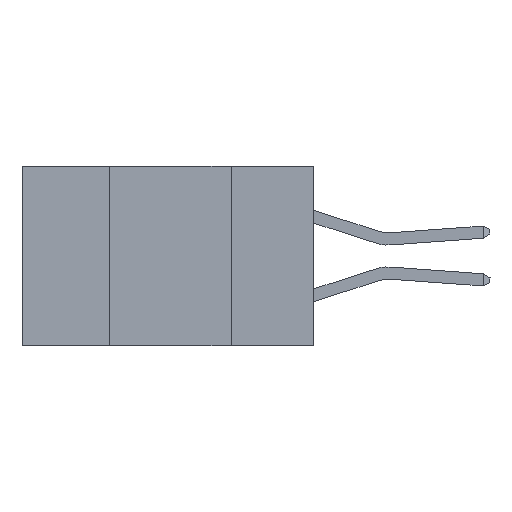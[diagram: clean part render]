
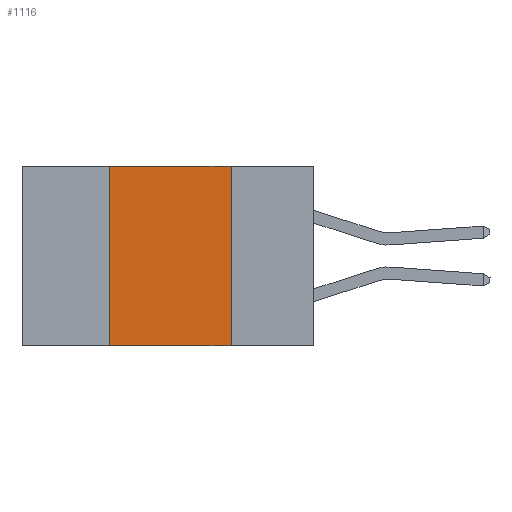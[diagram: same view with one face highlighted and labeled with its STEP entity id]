
A CAD part, left-side view. The second image highlights one B-rep face of the part: STEP entity #1116.
In plain terms, the highlighted planar face has unit normal (-1, 0, 0).
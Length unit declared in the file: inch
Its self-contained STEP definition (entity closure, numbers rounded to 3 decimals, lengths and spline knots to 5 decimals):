
#257 = VERTEX_POINT ( 'NONE', #1028 ) ;
#342 = DIRECTION ( 'NONE',  ( 0., 0., -1. ) ) ;
#811 = FACE_OUTER_BOUND ( 'NONE', #4096, .T. ) ;
#956 = CARTESIAN_POINT ( 'NONE',  ( 0., 0.17, 0. ) ) ;
#1028 = CARTESIAN_POINT ( 'NONE',  ( 0., 0.42, -0.37 ) ) ;
#1116 = ADVANCED_FACE ( 'NONE', ( #811 ), #3273, .F. ) ;
#1811 = VECTOR ( 'NONE', #8453, 39.37008 ) ;
#1971 = ORIENTED_EDGE ( 'NONE', *, *, #2123, .F. ) ;
#2123 = EDGE_CURVE ( 'NONE', #13648, #8218, #11626, .T. ) ;
#2273 = EDGE_CURVE ( 'NONE', #8218, #4752, #3621, .T. ) ;
#2320 = EDGE_CURVE ( 'NONE', #257, #13648, #8511, .T. ) ;
#2339 = ORIENTED_EDGE ( 'NONE', *, *, #2320, .F. ) ;
#2341 = EDGE_CURVE ( 'NONE', #257, #4752, #10575, .T. ) ;
#2538 = VECTOR ( 'NONE', #8687, 39.37008 ) ;
#3273 = PLANE ( 'NONE',  #4331 ) ;
#3621 = LINE ( 'NONE', #9256, #11777 ) ;
#4096 = EDGE_LOOP ( 'NONE', ( #12920, #1971, #2339, #13459 ) ) ;
#4331 = AXIS2_PLACEMENT_3D ( 'NONE', #11544, #12778, #342 ) ;
#4654 = CARTESIAN_POINT ( 'NONE',  ( 0., 0.17, -0.37 ) ) ;
#4752 = VERTEX_POINT ( 'NONE', #4654 ) ;
#8218 = VERTEX_POINT ( 'NONE', #956 ) ;
#8438 = CARTESIAN_POINT ( 'NONE',  ( 0., 0.6, -0.37 ) ) ;
#8453 = DIRECTION ( 'NONE',  ( 0., -1., 0. ) ) ;
#8511 = LINE ( 'NONE', #8730, #2538 ) ;
#8687 = DIRECTION ( 'NONE',  ( 0., 0., 1. ) ) ;
#8730 = CARTESIAN_POINT ( 'NONE',  ( 0., 0.42, 0. ) ) ;
#8750 = CARTESIAN_POINT ( 'NONE',  ( 0., 0.42, 0. ) ) ;
#9256 = CARTESIAN_POINT ( 'NONE',  ( 0., 0.17, 0. ) ) ;
#9298 = DIRECTION ( 'NONE',  ( 0., 0., -1. ) ) ;
#9645 = VECTOR ( 'NONE', #10694, 39.37008 ) ;
#10575 = LINE ( 'NONE', #8438, #1811 ) ;
#10659 = CARTESIAN_POINT ( 'NONE',  ( 0., 0.6, 0. ) ) ;
#10694 = DIRECTION ( 'NONE',  ( 0., -1., 0. ) ) ;
#11544 = CARTESIAN_POINT ( 'NONE',  ( 0., 0.6, 0. ) ) ;
#11626 = LINE ( 'NONE', #10659, #9645 ) ;
#11777 = VECTOR ( 'NONE', #9298, 39.37008 ) ;
#12778 = DIRECTION ( 'NONE',  ( 1., 0., 0. ) ) ;
#12920 = ORIENTED_EDGE ( 'NONE', *, *, #2273, .F. ) ;
#13459 = ORIENTED_EDGE ( 'NONE', *, *, #2341, .T. ) ;
#13648 = VERTEX_POINT ( 'NONE', #8750 ) ;
